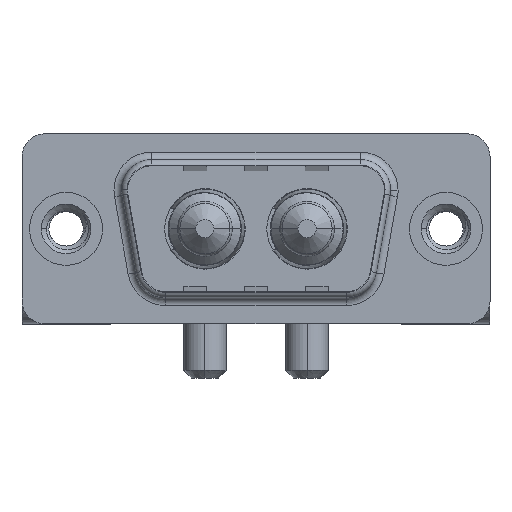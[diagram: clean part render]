
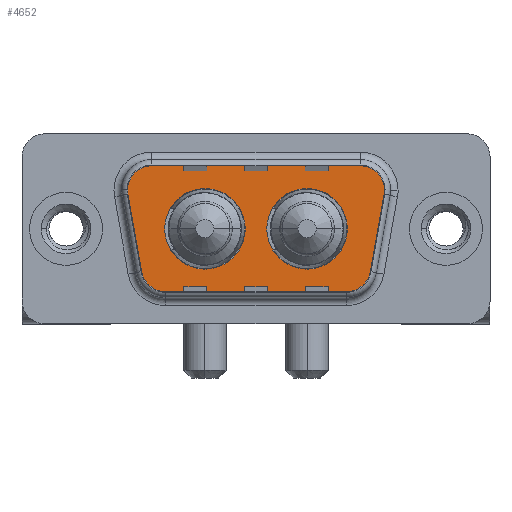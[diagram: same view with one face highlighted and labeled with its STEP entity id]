
A CAD part, top view. The second image highlights one B-rep face of the part: STEP entity #4652.
In plain terms, the highlighted planar face has unit normal (0, 0, 1).
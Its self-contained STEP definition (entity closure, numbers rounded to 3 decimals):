
#3 = VERTEX_POINT ( 'NONE', #3214 ) ;
#48 = CARTESIAN_POINT ( 'NONE',  ( 6.49, 0., 0. ) ) ;
#66 = CIRCLE ( 'NONE', #1669, 2. ) ;
#317 = CARTESIAN_POINT ( 'NONE',  ( 9.14, 0., 0. ) ) ;
#432 = CARTESIAN_POINT ( 'NONE',  ( 18.541, -2.9, 0. ) ) ;
#459 = CARTESIAN_POINT ( 'NONE',  ( 19.564, 2.9, 0. ) ) ;
#467 = CARTESIAN_POINT ( 'NONE',  ( 5.436, 4.9, 0. ) ) ;
#878 = CIRCLE ( 'NONE', #12216, 2.65 ) ;
#971 = ORIENTED_EDGE ( 'NONE', *, *, #1727, .T. ) ;
#1009 = VECTOR ( 'NONE', #3059, 1000. ) ;
#1285 = EDGE_LOOP ( 'NONE', ( #8686, #3229, #8958, #10299, #5568, #2611, #9691, #971, #10700 ) ) ;
#1287 = CARTESIAN_POINT ( 'NONE',  ( 11.79, 0., 0. ) ) ;
#1602 = DIRECTION ( 'NONE',  ( 0.174, -0.985, 0. ) ) ;
#1669 = AXIS2_PLACEMENT_3D ( 'NONE', #459, #9878, #6174 ) ;
#1727 = EDGE_CURVE ( 'NONE', #3, #11055, #8257, .T. ) ;
#1922 = DIRECTION ( 'NONE',  ( 0., 0., 1. ) ) ;
#1957 = ORIENTED_EDGE ( 'NONE', *, *, #3438, .F. ) ;
#2003 = DIRECTION ( 'NONE',  ( 0., 0., 1. ) ) ;
#2112 = FACE_BOUND ( 'NONE', #7235, .T. ) ;
#2181 = DIRECTION ( 'NONE',  ( 0., 0., 1. ) ) ;
#2201 = DIRECTION ( 'NONE',  ( 1., 0., 0. ) ) ;
#2212 = DIRECTION ( 'NONE',  ( 1., 0., 0. ) ) ;
#2389 = CARTESIAN_POINT ( 'NONE',  ( 21.534, 2.553, 0. ) ) ;
#2591 = ORIENTED_EDGE ( 'NONE', *, *, #9019, .F. ) ;
#2611 = ORIENTED_EDGE ( 'NONE', *, *, #5174, .T. ) ;
#2615 = AXIS2_PLACEMENT_3D ( 'NONE', #10463, #1922, #6772 ) ;
#2664 = DIRECTION ( 'NONE',  ( 0., 0., 1. ) ) ;
#2703 = CIRCLE ( 'NONE', #2886, 2. ) ;
#2886 = AXIS2_PLACEMENT_3D ( 'NONE', #432, #2664, #8379 ) ;
#2891 = AXIS2_PLACEMENT_3D ( 'NONE', #4332, #9270, #11945 ) ;
#2927 = DIRECTION ( 'NONE',  ( -1., 0., 0. ) ) ;
#2996 = EDGE_CURVE ( 'NONE', #11356, #5134, #2703, .T. ) ;
#3031 = DIRECTION ( 'NONE',  ( 1., 0., 0. ) ) ;
#3059 = DIRECTION ( 'NONE',  ( 1., 0., 0. ) ) ;
#3214 = CARTESIAN_POINT ( 'NONE',  ( 4.489, -3.247, 0. ) ) ;
#3229 = ORIENTED_EDGE ( 'NONE', *, *, #5949, .T. ) ;
#3349 = EDGE_CURVE ( 'NONE', #8159, #7418, #66, .T. ) ;
#3360 = CARTESIAN_POINT ( 'NONE',  ( 18.541, -4.9, 0. ) ) ;
#3363 = CARTESIAN_POINT ( 'NONE',  ( 18.51, 0., 0. ) ) ;
#3438 = EDGE_CURVE ( 'NONE', #9254, #4131, #878, .T. ) ;
#3648 = CARTESIAN_POINT ( 'NONE',  ( 21.564, 2.9, 0. ) ) ;
#3832 = CARTESIAN_POINT ( 'NONE',  ( 20.511, -3.247, 0. ) ) ;
#4131 = VERTEX_POINT ( 'NONE', #6016 ) ;
#4332 = CARTESIAN_POINT ( 'NONE',  ( 6.459, -2.9, 0. ) ) ;
#4343 = CIRCLE ( 'NONE', #9720, 2. ) ;
#4652 = ADVANCED_FACE ( 'NONE', ( #2112, #7825, #4896 ), #4831, .T. ) ;
#4831 = PLANE ( 'NONE',  #7125 ) ;
#4896 = FACE_OUTER_BOUND ( 'NONE', #1285, .T. ) ;
#4968 = CARTESIAN_POINT ( 'NONE',  ( 19.564, 2.9, 0. ) ) ;
#5015 = AXIS2_PLACEMENT_3D ( 'NONE', #4968, #2181, #8781 ) ;
#5134 = VERTEX_POINT ( 'NONE', #3832 ) ;
#5174 = EDGE_CURVE ( 'NONE', #9708, #10441, #4343, .T. ) ;
#5432 = DIRECTION ( 'NONE',  ( 0.174, 0.985, 0. ) ) ;
#5568 = ORIENTED_EDGE ( 'NONE', *, *, #11021, .T. ) ;
#5645 = ORIENTED_EDGE ( 'NONE', *, *, #7983, .F. ) ;
#5651 = CARTESIAN_POINT ( 'NONE',  ( 3.466, 2.553, 0. ) ) ;
#5918 = VECTOR ( 'NONE', #5432, 1000. ) ;
#5949 = EDGE_CURVE ( 'NONE', #5134, #8159, #8253, .T. ) ;
#6016 = CARTESIAN_POINT ( 'NONE',  ( 13.21, 0., 0. ) ) ;
#6174 = DIRECTION ( 'NONE',  ( -1., 0., 0. ) ) ;
#6270 = EDGE_CURVE ( 'NONE', #4131, #9254, #10531, .T. ) ;
#6417 = DIRECTION ( 'NONE',  ( 1., 0., 0. ) ) ;
#6515 = ORIENTED_EDGE ( 'NONE', *, *, #6270, .F. ) ;
#6678 = DIRECTION ( 'NONE',  ( 0., 0., 1. ) ) ;
#6704 = CARTESIAN_POINT ( 'NONE',  ( 6.459, -4.9, 0. ) ) ;
#6772 = DIRECTION ( 'NONE',  ( 1., 0., 0. ) ) ;
#6951 = AXIS2_PLACEMENT_3D ( 'NONE', #317, #2003, #2201 ) ;
#7024 = VECTOR ( 'NONE', #1602, 1000. ) ;
#7125 = AXIS2_PLACEMENT_3D ( 'NONE', #9772, #10572, #11636 ) ;
#7126 = VERTEX_POINT ( 'NONE', #1287 ) ;
#7220 = VECTOR ( 'NONE', #2927, 1000. ) ;
#7235 = EDGE_LOOP ( 'NONE', ( #1957, #6515 ) ) ;
#7245 = CARTESIAN_POINT ( 'NONE',  ( 15.86, 0., 0. ) ) ;
#7412 = LINE ( 'NONE', #9527, #7220 ) ;
#7418 = VERTEX_POINT ( 'NONE', #3648 ) ;
#7712 = CARTESIAN_POINT ( 'NONE',  ( 6.459, -4.9, 0. ) ) ;
#7825 = FACE_BOUND ( 'NONE', #12064, .T. ) ;
#7953 = CIRCLE ( 'NONE', #6951, 2.65 ) ;
#7983 = EDGE_CURVE ( 'NONE', #7126, #11183, #7953, .T. ) ;
#8159 = VERTEX_POINT ( 'NONE', #2389 ) ;
#8253 = LINE ( 'NONE', #12055, #5918 ) ;
#8257 = CIRCLE ( 'NONE', #2891, 2. ) ;
#8269 = LINE ( 'NONE', #8617, #7024 ) ;
#8379 = DIRECTION ( 'NONE',  ( 1., 0., 0. ) ) ;
#8617 = CARTESIAN_POINT ( 'NONE',  ( 3.466, 2.553, 0. ) ) ;
#8676 = DIRECTION ( 'NONE',  ( 0., 0., 1. ) ) ;
#8686 = ORIENTED_EDGE ( 'NONE', *, *, #2996, .T. ) ;
#8781 = DIRECTION ( 'NONE',  ( -1., 0., 0. ) ) ;
#8849 = LINE ( 'NONE', #6704, #1009 ) ;
#8958 = ORIENTED_EDGE ( 'NONE', *, *, #3349, .T. ) ;
#8984 = EDGE_CURVE ( 'NONE', #11055, #11356, #8849, .T. ) ;
#9019 = EDGE_CURVE ( 'NONE', #11183, #7126, #10361, .T. ) ;
#9149 = AXIS2_PLACEMENT_3D ( 'NONE', #9614, #8676, #2212 ) ;
#9254 = VERTEX_POINT ( 'NONE', #3363 ) ;
#9270 = DIRECTION ( 'NONE',  ( 0., 0., 1. ) ) ;
#9304 = CARTESIAN_POINT ( 'NONE',  ( 19.564, 4.9, 0. ) ) ;
#9527 = CARTESIAN_POINT ( 'NONE',  ( 5.436, 4.9, 0. ) ) ;
#9614 = CARTESIAN_POINT ( 'NONE',  ( 15.86, 0., 0. ) ) ;
#9691 = ORIENTED_EDGE ( 'NONE', *, *, #11496, .T. ) ;
#9708 = VERTEX_POINT ( 'NONE', #467 ) ;
#9720 = AXIS2_PLACEMENT_3D ( 'NONE', #10373, #6678, #3031 ) ;
#9772 = CARTESIAN_POINT ( 'NONE',  ( 18.541, -2.9, 0. ) ) ;
#9878 = DIRECTION ( 'NONE',  ( 0., 0., 1. ) ) ;
#10299 = ORIENTED_EDGE ( 'NONE', *, *, #11167, .T. ) ;
#10361 = CIRCLE ( 'NONE', #2615, 2.65 ) ;
#10373 = CARTESIAN_POINT ( 'NONE',  ( 5.436, 2.9, 0. ) ) ;
#10441 = VERTEX_POINT ( 'NONE', #5651 ) ;
#10463 = CARTESIAN_POINT ( 'NONE',  ( 9.14, 0., 0. ) ) ;
#10531 = CIRCLE ( 'NONE', #9149, 2.65 ) ;
#10572 = DIRECTION ( 'NONE',  ( 0., 0., 1. ) ) ;
#10700 = ORIENTED_EDGE ( 'NONE', *, *, #8984, .T. ) ;
#11021 = EDGE_CURVE ( 'NONE', #11948, #9708, #7412, .T. ) ;
#11055 = VERTEX_POINT ( 'NONE', #7712 ) ;
#11166 = DIRECTION ( 'NONE',  ( 0., 0., 1. ) ) ;
#11167 = EDGE_CURVE ( 'NONE', #7418, #11948, #11391, .T. ) ;
#11183 = VERTEX_POINT ( 'NONE', #48 ) ;
#11356 = VERTEX_POINT ( 'NONE', #3360 ) ;
#11391 = CIRCLE ( 'NONE', #5015, 2. ) ;
#11496 = EDGE_CURVE ( 'NONE', #10441, #3, #8269, .T. ) ;
#11636 = DIRECTION ( 'NONE',  ( 1., 0., 0. ) ) ;
#11945 = DIRECTION ( 'NONE',  ( -1., 0., 0. ) ) ;
#11948 = VERTEX_POINT ( 'NONE', #9304 ) ;
#12055 = CARTESIAN_POINT ( 'NONE',  ( 21.534, 2.553, 0. ) ) ;
#12064 = EDGE_LOOP ( 'NONE', ( #5645, #2591 ) ) ;
#12216 = AXIS2_PLACEMENT_3D ( 'NONE', #7245, #11166, #6417 ) ;
